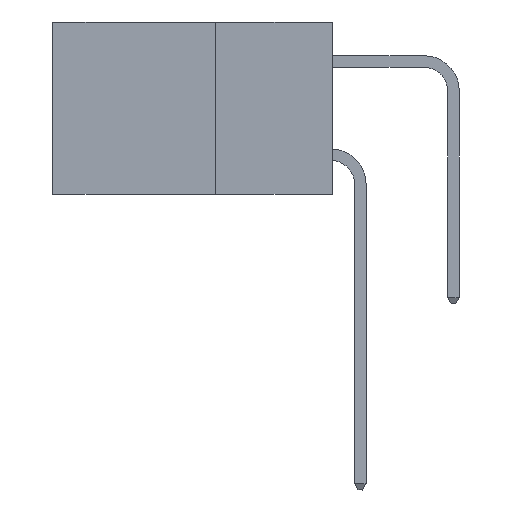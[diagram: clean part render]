
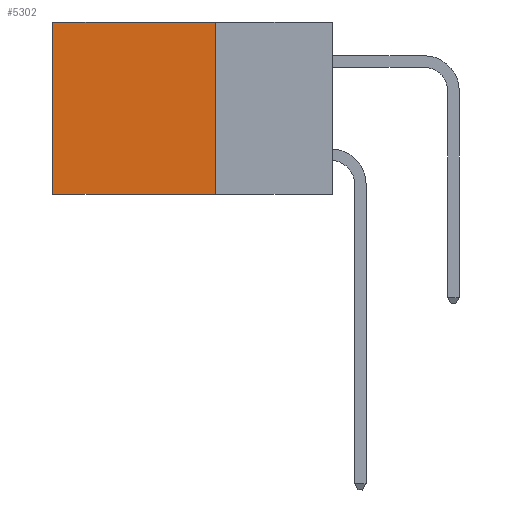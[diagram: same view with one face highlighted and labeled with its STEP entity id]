
A CAD part, left-side view. The second image highlights one B-rep face of the part: STEP entity #5302.
In plain terms, the highlighted planar face has unit normal (-1, 0, 0).
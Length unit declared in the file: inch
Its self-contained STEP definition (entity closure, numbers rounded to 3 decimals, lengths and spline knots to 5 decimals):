
#106 = EDGE_CURVE ( 'NONE', #10425, #778, #11136, .T. ) ;
#186 = CARTESIAN_POINT ( 'NONE',  ( 0.298, 0.25, 0. ) ) ;
#303 = FACE_OUTER_BOUND ( 'NONE', #10365, .T. ) ;
#449 = VERTEX_POINT ( 'NONE', #1542 ) ;
#778 = VERTEX_POINT ( 'NONE', #4435 ) ;
#1221 = ORIENTED_EDGE ( 'NONE', *, *, #106, .F. ) ;
#1259 = LINE ( 'NONE', #9421, #6520 ) ;
#1477 = VERTEX_POINT ( 'NONE', #5840 ) ;
#1542 = CARTESIAN_POINT ( 'NONE',  ( 0.298, 0.6, -0.37 ) ) ;
#2290 = ORIENTED_EDGE ( 'NONE', *, *, #10918, .T. ) ;
#2508 = DIRECTION ( 'NONE',  ( 0., 0., -1. ) ) ;
#2868 = VECTOR ( 'NONE', #9947, 39.37008 ) ;
#3691 = CARTESIAN_POINT ( 'NONE',  ( 0.298, 0.25, 0. ) ) ;
#4265 = ORIENTED_EDGE ( 'NONE', *, *, #10562, .F. ) ;
#4435 = CARTESIAN_POINT ( 'NONE',  ( 0.298, 0.25, -0.37 ) ) ;
#5062 = CARTESIAN_POINT ( 'NONE',  ( 0.298, 0.25, 0. ) ) ;
#5302 = ADVANCED_FACE ( 'NONE', ( #303 ), #12564, .F. ) ;
#5840 = CARTESIAN_POINT ( 'NONE',  ( 0.298, 0.6, 0. ) ) ;
#5899 = VECTOR ( 'NONE', #2508, 39.37008 ) ;
#6520 = VECTOR ( 'NONE', #12643, 39.37008 ) ;
#6790 = CARTESIAN_POINT ( 'NONE',  ( 0.298, 0.6, 0. ) ) ;
#6872 = CARTESIAN_POINT ( 'NONE',  ( 0.298, 0.25, 0. ) ) ;
#7500 = DIRECTION ( 'NONE',  ( 0., 1., 0. ) ) ;
#7592 = EDGE_CURVE ( 'NONE', #10425, #1477, #8257, .T. ) ;
#8257 = LINE ( 'NONE', #186, #11068 ) ;
#8784 = DIRECTION ( 'NONE',  ( 1., 0., 0. ) ) ;
#8803 = LINE ( 'NONE', #6790, #2868 ) ;
#9421 = CARTESIAN_POINT ( 'NONE',  ( 0.298, 0.25, -0.37 ) ) ;
#9947 = DIRECTION ( 'NONE',  ( 0., 0., -1. ) ) ;
#10261 = ORIENTED_EDGE ( 'NONE', *, *, #7592, .T. ) ;
#10365 = EDGE_LOOP ( 'NONE', ( #2290, #4265, #1221, #10261 ) ) ;
#10425 = VERTEX_POINT ( 'NONE', #5062 ) ;
#10562 = EDGE_CURVE ( 'NONE', #778, #449, #1259, .T. ) ;
#10918 = EDGE_CURVE ( 'NONE', #1477, #449, #8803, .T. ) ;
#11068 = VECTOR ( 'NONE', #7500, 39.37008 ) ;
#11136 = LINE ( 'NONE', #6872, #5899 ) ;
#12564 = PLANE ( 'NONE',  #12713 ) ;
#12643 = DIRECTION ( 'NONE',  ( 0., 1., 0. ) ) ;
#12713 = AXIS2_PLACEMENT_3D ( 'NONE', #3691, #8784, #13131 ) ;
#13131 = DIRECTION ( 'NONE',  ( 0., 0., -1. ) ) ;
